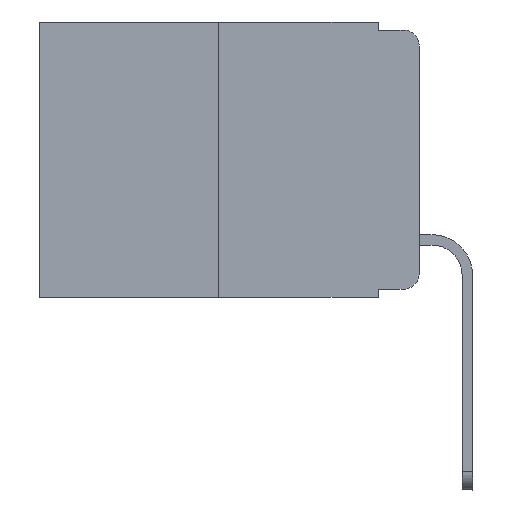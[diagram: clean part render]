
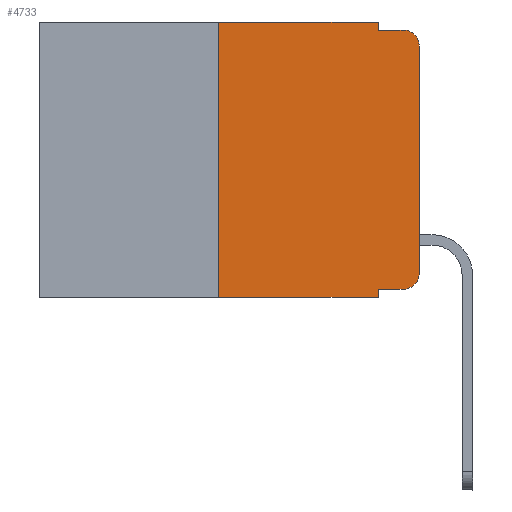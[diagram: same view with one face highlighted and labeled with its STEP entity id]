
A CAD part, left-side view. The second image highlights one B-rep face of the part: STEP entity #4733.
In plain terms, the highlighted planar face has unit normal (-1, 0, 0).
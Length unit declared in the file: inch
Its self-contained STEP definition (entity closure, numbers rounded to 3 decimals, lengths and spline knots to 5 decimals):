
#76 = DIRECTION ( 'NONE',  ( 0., 0., 1. ) ) ;
#199 = VERTEX_POINT ( 'NONE', #9944 ) ;
#258 = ORIENTED_EDGE ( 'NONE', *, *, #9061, .F. ) ;
#298 = EDGE_CURVE ( 'NONE', #7072, #11136, #5519, .T. ) ;
#540 = CARTESIAN_POINT ( 'NONE',  ( 0., 0., -0.03 ) ) ;
#707 = VERTEX_POINT ( 'NONE', #11324 ) ;
#788 = ORIENTED_EDGE ( 'NONE', *, *, #11189, .T. ) ;
#1043 = CARTESIAN_POINT ( 'NONE',  ( 0., 0.473, -0.343 ) ) ;
#1458 = CARTESIAN_POINT ( 'NONE',  ( 0., 0.051, -0.333 ) ) ;
#1696 = CARTESIAN_POINT ( 'NONE',  ( 0., 0.051, 0. ) ) ;
#1790 = FACE_OUTER_BOUND ( 'NONE', #8914, .T. ) ;
#1934 = DIRECTION ( 'NONE',  ( 0., -1., 0. ) ) ;
#1972 = PLANE ( 'NONE',  #9594 ) ;
#2094 = VECTOR ( 'NONE', #6961, 39.37008 ) ;
#2804 = VERTEX_POINT ( 'NONE', #7933 ) ;
#3076 = VERTEX_POINT ( 'NONE', #4842 ) ;
#3083 = ORIENTED_EDGE ( 'NONE', *, *, #7902, .F. ) ;
#3140 = CARTESIAN_POINT ( 'NONE',  ( 0., 0.051, 0. ) ) ;
#3372 = CARTESIAN_POINT ( 'NONE',  ( 0., 0.02, -0.313 ) ) ;
#3622 = EDGE_CURVE ( 'NONE', #10632, #7072, #10001, .T. ) ;
#3665 = DIRECTION ( 'NONE',  ( 0., 0., -1. ) ) ;
#3763 = VERTEX_POINT ( 'NONE', #1696 ) ;
#4060 = VECTOR ( 'NONE', #76, 39.37008 ) ;
#4123 = ORIENTED_EDGE ( 'NONE', *, *, #8971, .F. ) ;
#4390 = VECTOR ( 'NONE', #11908, 39.37008 ) ;
#4596 = LINE ( 'NONE', #12201, #5490 ) ;
#4641 = LINE ( 'NONE', #3140, #2094 ) ;
#4733 = ADVANCED_FACE ( 'NONE', ( #1790 ), #1972, .F. ) ;
#4798 = LINE ( 'NONE', #8629, #4060 ) ;
#4812 = DIRECTION ( 'NONE',  ( -1., 0., 0. ) ) ;
#4842 = CARTESIAN_POINT ( 'NONE',  ( 0., 0.051, -0.343 ) ) ;
#4938 = ORIENTED_EDGE ( 'NONE', *, *, #5293, .T. ) ;
#4995 = LINE ( 'NONE', #8007, #8864 ) ;
#5015 = VECTOR ( 'NONE', #11822, 39.37008 ) ;
#5094 = VECTOR ( 'NONE', #1934, 39.37008 ) ;
#5126 = ORIENTED_EDGE ( 'NONE', *, *, #7844, .F. ) ;
#5147 = ORIENTED_EDGE ( 'NONE', *, *, #5994, .T. ) ;
#5259 = DIRECTION ( 'NONE',  ( -1., 0., 0. ) ) ;
#5293 = EDGE_CURVE ( 'NONE', #11136, #9725, #6059, .T. ) ;
#5490 = VECTOR ( 'NONE', #3665, 39.37008 ) ;
#5519 = CIRCLE ( 'NONE', #10712, 0.02 ) ;
#5782 = ORIENTED_EDGE ( 'NONE', *, *, #8626, .F. ) ;
#5835 = CARTESIAN_POINT ( 'NONE',  ( 0., 0.02, -0.03 ) ) ;
#5994 = EDGE_CURVE ( 'NONE', #9725, #199, #9024, .T. ) ;
#6059 = LINE ( 'NONE', #8235, #5015 ) ;
#6089 = CARTESIAN_POINT ( 'NONE',  ( 0., 0., -0.313 ) ) ;
#6961 = DIRECTION ( 'NONE',  ( 0., 0., -1. ) ) ;
#7072 = VERTEX_POINT ( 'NONE', #9149 ) ;
#7695 = VECTOR ( 'NONE', #9012, 39.37008 ) ;
#7745 = ORIENTED_EDGE ( 'NONE', *, *, #3622, .T. ) ;
#7844 = EDGE_CURVE ( 'NONE', #707, #11992, #4798, .T. ) ;
#7902 = EDGE_CURVE ( 'NONE', #2804, #199, #4995, .T. ) ;
#7933 = CARTESIAN_POINT ( 'NONE',  ( 0., 0.051, -0.01 ) ) ;
#8007 = CARTESIAN_POINT ( 'NONE',  ( 0., 0.051, -0.01 ) ) ;
#8235 = CARTESIAN_POINT ( 'NONE',  ( 0., 0., 0. ) ) ;
#8626 = EDGE_CURVE ( 'NONE', #10632, #3076, #4641, .T. ) ;
#8629 = CARTESIAN_POINT ( 'NONE',  ( 0., 0.25, 0. ) ) ;
#8864 = VECTOR ( 'NONE', #9064, 39.37008 ) ;
#8914 = EDGE_LOOP ( 'NONE', ( #4938, #5147, #3083, #258, #4123, #5126, #788, #5782, #7745, #9086 ) ) ;
#8971 = EDGE_CURVE ( 'NONE', #11992, #3763, #10233, .T. ) ;
#9012 = DIRECTION ( 'NONE',  ( 0., -1., 0. ) ) ;
#9024 = CIRCLE ( 'NONE', #10021, 0.02 ) ;
#9061 = EDGE_CURVE ( 'NONE', #3763, #2804, #4596, .T. ) ;
#9064 = DIRECTION ( 'NONE',  ( 0., -1., 0. ) ) ;
#9086 = ORIENTED_EDGE ( 'NONE', *, *, #298, .T. ) ;
#9149 = CARTESIAN_POINT ( 'NONE',  ( 0., 0.02, -0.333 ) ) ;
#9540 = CARTESIAN_POINT ( 'NONE',  ( 0., 0.051, -0.333 ) ) ;
#9594 = AXIS2_PLACEMENT_3D ( 'NONE', #12242, #10272, #11200 ) ;
#9643 = LINE ( 'NONE', #1043, #7695 ) ;
#9663 = CARTESIAN_POINT ( 'NONE',  ( 0., 0.25, 0. ) ) ;
#9725 = VERTEX_POINT ( 'NONE', #540 ) ;
#9944 = CARTESIAN_POINT ( 'NONE',  ( 0., 0.02, -0.01 ) ) ;
#10001 = LINE ( 'NONE', #1458, #4390 ) ;
#10021 = AXIS2_PLACEMENT_3D ( 'NONE', #5835, #4812, #10516 ) ;
#10124 = DIRECTION ( 'NONE',  ( 0., 0., -1. ) ) ;
#10233 = LINE ( 'NONE', #11158, #5094 ) ;
#10272 = DIRECTION ( 'NONE',  ( 1., 0., 0. ) ) ;
#10516 = DIRECTION ( 'NONE',  ( 0., 0., -1. ) ) ;
#10632 = VERTEX_POINT ( 'NONE', #9540 ) ;
#10712 = AXIS2_PLACEMENT_3D ( 'NONE', #3372, #5259, #10124 ) ;
#11136 = VERTEX_POINT ( 'NONE', #6089 ) ;
#11158 = CARTESIAN_POINT ( 'NONE',  ( 0., 0.473, 0. ) ) ;
#11189 = EDGE_CURVE ( 'NONE', #707, #3076, #9643, .T. ) ;
#11200 = DIRECTION ( 'NONE',  ( 0., 0., -1. ) ) ;
#11324 = CARTESIAN_POINT ( 'NONE',  ( 0., 0.25, -0.343 ) ) ;
#11822 = DIRECTION ( 'NONE',  ( 0., 0., 1. ) ) ;
#11908 = DIRECTION ( 'NONE',  ( 0., -1., 0. ) ) ;
#11992 = VERTEX_POINT ( 'NONE', #9663 ) ;
#12201 = CARTESIAN_POINT ( 'NONE',  ( 0., 0.051, 0. ) ) ;
#12242 = CARTESIAN_POINT ( 'NONE',  ( 0., 0.473, 0. ) ) ;
